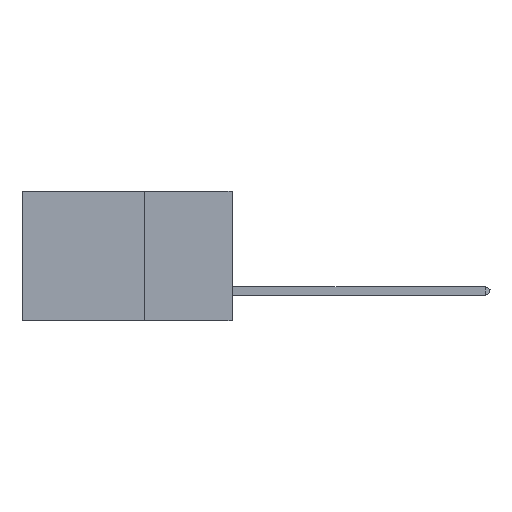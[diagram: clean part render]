
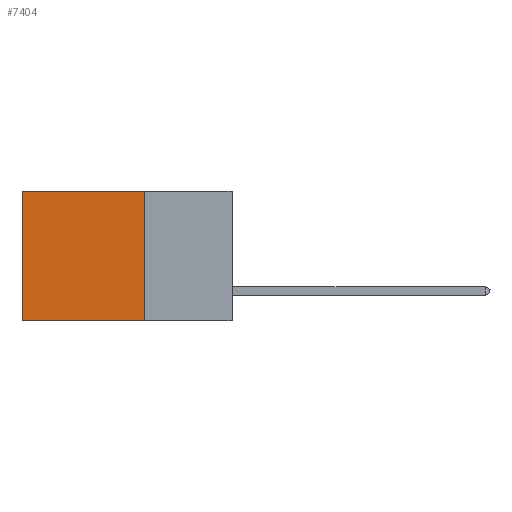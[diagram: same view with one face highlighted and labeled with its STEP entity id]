
A CAD part, left-side view. The second image highlights one B-rep face of the part: STEP entity #7404.
In plain terms, the highlighted planar face has unit normal (-1, 0, 0).
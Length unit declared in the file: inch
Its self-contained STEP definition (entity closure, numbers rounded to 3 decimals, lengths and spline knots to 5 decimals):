
#173 = DIRECTION ( 'NONE',  ( 1., 0., 0. ) ) ;
#645 = DIRECTION ( 'NONE',  ( 0., 0., -1. ) ) ;
#1385 = CARTESIAN_POINT ( 'NONE',  ( 0.2875, 0.6, 0. ) ) ;
#2054 = AXIS2_PLACEMENT_3D ( 'NONE', #26626, #173, #22080 ) ;
#2325 = EDGE_CURVE ( 'NONE', #19660, #25059, #18379, .T. ) ;
#2647 = VERTEX_POINT ( 'NONE', #3511 ) ;
#2908 = EDGE_LOOP ( 'NONE', ( #9971, #7325, #10888, #13959 ) ) ;
#3511 = CARTESIAN_POINT ( 'NONE',  ( 0.2875, 0.25, -0.37 ) ) ;
#4602 = VERTEX_POINT ( 'NONE', #27795 ) ;
#5462 = EDGE_CURVE ( 'NONE', #19660, #2647, #27725, .T. ) ;
#6293 = LINE ( 'NONE', #22266, #17228 ) ;
#6420 = DIRECTION ( 'NONE',  ( 0., 0., -1. ) ) ;
#7325 = ORIENTED_EDGE ( 'NONE', *, *, #23236, .F. ) ;
#7404 = ADVANCED_FACE ( 'NONE', ( #17063 ), #17058, .F. ) ;
#8560 = CARTESIAN_POINT ( 'NONE',  ( 0.2875, 0.25, 0. ) ) ;
#9311 = CARTESIAN_POINT ( 'NONE',  ( 0.2875, 0.25, -0.37 ) ) ;
#9971 = ORIENTED_EDGE ( 'NONE', *, *, #15108, .T. ) ;
#10888 = ORIENTED_EDGE ( 'NONE', *, *, #5462, .F. ) ;
#11827 = VECTOR ( 'NONE', #24882, 39.37008 ) ;
#13959 = ORIENTED_EDGE ( 'NONE', *, *, #2325, .T. ) ;
#15108 = EDGE_CURVE ( 'NONE', #25059, #4602, #6293, .T. ) ;
#16706 = CARTESIAN_POINT ( 'NONE',  ( 0.2875, 0.25, 0. ) ) ;
#17058 = PLANE ( 'NONE',  #2054 ) ;
#17063 = FACE_OUTER_BOUND ( 'NONE', #2908, .T. ) ;
#17228 = VECTOR ( 'NONE', #645, 39.37008 ) ;
#17574 = LINE ( 'NONE', #9311, #11827 ) ;
#18379 = LINE ( 'NONE', #16706, #25151 ) ;
#19660 = VERTEX_POINT ( 'NONE', #22766 ) ;
#22080 = DIRECTION ( 'NONE',  ( 0., 0., -1. ) ) ;
#22266 = CARTESIAN_POINT ( 'NONE',  ( 0.2875, 0.6, 0. ) ) ;
#22766 = CARTESIAN_POINT ( 'NONE',  ( 0.2875, 0.25, 0. ) ) ;
#23236 = EDGE_CURVE ( 'NONE', #2647, #4602, #17574, .T. ) ;
#23265 = DIRECTION ( 'NONE',  ( 0., 1., 0. ) ) ;
#24882 = DIRECTION ( 'NONE',  ( 0., 1., 0. ) ) ;
#25059 = VERTEX_POINT ( 'NONE', #1385 ) ;
#25151 = VECTOR ( 'NONE', #23265, 39.37008 ) ;
#26626 = CARTESIAN_POINT ( 'NONE',  ( 0.2875, 0.25, 0. ) ) ;
#27379 = VECTOR ( 'NONE', #6420, 39.37008 ) ;
#27725 = LINE ( 'NONE', #8560, #27379 ) ;
#27795 = CARTESIAN_POINT ( 'NONE',  ( 0.2875, 0.6, -0.37 ) ) ;
